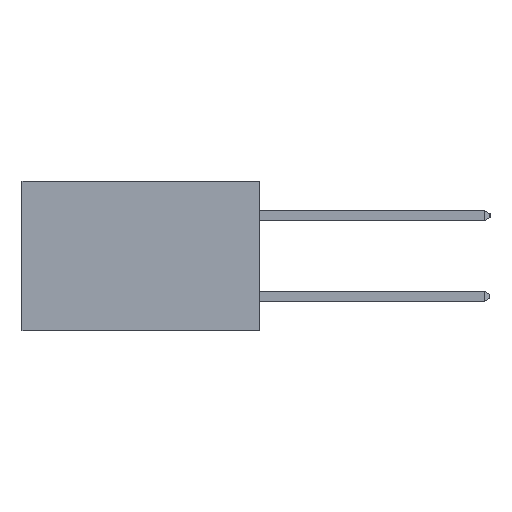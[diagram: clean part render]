
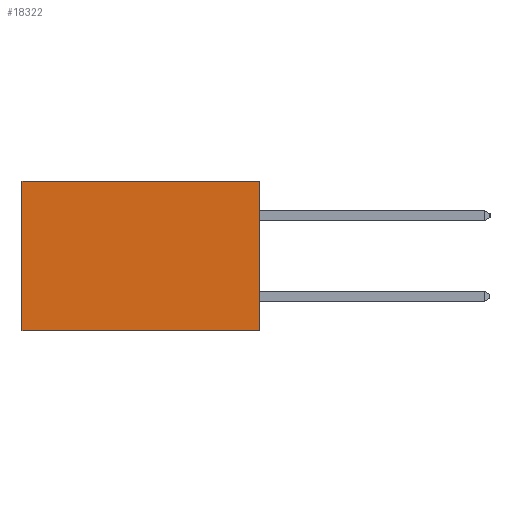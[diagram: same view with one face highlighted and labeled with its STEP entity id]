
A CAD part, left-side view. The second image highlights one B-rep face of the part: STEP entity #18322.
In plain terms, the highlighted planar face has unit normal (-1, 0, 0).
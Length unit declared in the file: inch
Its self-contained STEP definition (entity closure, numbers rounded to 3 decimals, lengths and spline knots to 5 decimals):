
#748 = EDGE_CURVE ( 'NONE', #8833, #18098, #5637, .T. ) ;
#1469 = DIRECTION ( 'NONE',  ( 0., 0., -1. ) ) ;
#1637 = CARTESIAN_POINT ( 'NONE',  ( 0.277, 0.59, -0.37 ) ) ;
#2204 = ORIENTED_EDGE ( 'NONE', *, *, #16829, .T. ) ;
#2249 = VERTEX_POINT ( 'NONE', #7882 ) ;
#2616 = DIRECTION ( 'NONE',  ( 0., 1., 0. ) ) ;
#2633 = ORIENTED_EDGE ( 'NONE', *, *, #11601, .T. ) ;
#5075 = VECTOR ( 'NONE', #17299, 39.37008 ) ;
#5637 = LINE ( 'NONE', #17135, #5075 ) ;
#6454 = AXIS2_PLACEMENT_3D ( 'NONE', #7910, #20325, #9694 ) ;
#6867 = ORIENTED_EDGE ( 'NONE', *, *, #748, .F. ) ;
#7088 = VECTOR ( 'NONE', #2616, 39.37008 ) ;
#7238 = ORIENTED_EDGE ( 'NONE', *, *, #9245, .F. ) ;
#7882 = CARTESIAN_POINT ( 'NONE',  ( 0.277, 0., 0. ) ) ;
#7910 = CARTESIAN_POINT ( 'NONE',  ( 0.277, 0., -0.37 ) ) ;
#8302 = EDGE_LOOP ( 'NONE', ( #2204, #6867, #7238, #2633 ) ) ;
#8833 = VERTEX_POINT ( 'NONE', #12077 ) ;
#9245 = EDGE_CURVE ( 'NONE', #2249, #8833, #18329, .T. ) ;
#9694 = DIRECTION ( 'NONE',  ( 0., 0., -1. ) ) ;
#11269 = LINE ( 'NONE', #15160, #7088 ) ;
#11296 = DIRECTION ( 'NONE',  ( 0., 0., -1. ) ) ;
#11601 = EDGE_CURVE ( 'NONE', #2249, #18449, #11269, .T. ) ;
#12077 = CARTESIAN_POINT ( 'NONE',  ( 0.277, 0., -0.37 ) ) ;
#13330 = VECTOR ( 'NONE', #1469, 39.37008 ) ;
#13543 = VECTOR ( 'NONE', #11296, 39.37008 ) ;
#13897 = LINE ( 'NONE', #22766, #13330 ) ;
#14113 = FACE_OUTER_BOUND ( 'NONE', #8302, .T. ) ;
#15160 = CARTESIAN_POINT ( 'NONE',  ( 0.277, 0., 0. ) ) ;
#15247 = CARTESIAN_POINT ( 'NONE',  ( 0.277, 0.59, 0. ) ) ;
#16829 = EDGE_CURVE ( 'NONE', #18449, #18098, #13897, .T. ) ;
#17135 = CARTESIAN_POINT ( 'NONE',  ( 0.277, 0., -0.37 ) ) ;
#17299 = DIRECTION ( 'NONE',  ( 0., 1., 0. ) ) ;
#18098 = VERTEX_POINT ( 'NONE', #1637 ) ;
#18322 = ADVANCED_FACE ( 'NONE', ( #14113 ), #18541, .F. ) ;
#18329 = LINE ( 'NONE', #20219, #13543 ) ;
#18449 = VERTEX_POINT ( 'NONE', #15247 ) ;
#18541 = PLANE ( 'NONE',  #6454 ) ;
#20219 = CARTESIAN_POINT ( 'NONE',  ( 0.277, 0., -0.37 ) ) ;
#20325 = DIRECTION ( 'NONE',  ( 1., 0., 0. ) ) ;
#22766 = CARTESIAN_POINT ( 'NONE',  ( 0.277, 0.59, -0.37 ) ) ;
